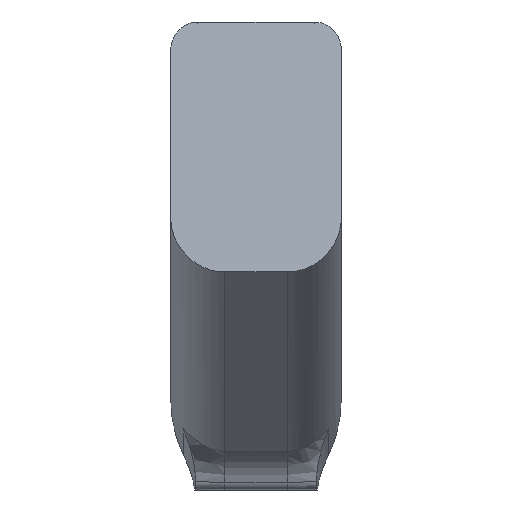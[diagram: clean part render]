
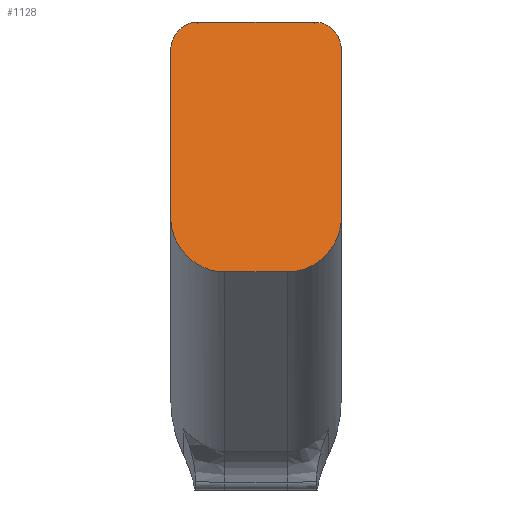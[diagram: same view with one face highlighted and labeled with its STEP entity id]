
A CAD part, front view. The second image highlights one B-rep face of the part: STEP entity #1128.
In plain terms, the highlighted planar face has unit normal (0, -0.978, 0.208).
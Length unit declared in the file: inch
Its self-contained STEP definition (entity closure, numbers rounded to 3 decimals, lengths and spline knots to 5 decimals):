
#7 = CARTESIAN_POINT ( 'NONE',  ( -0.22441, -2.64884, 0.92841 ) ) ;
#8 = CARTESIAN_POINT ( 'NONE',  ( -0.45503, -2.64884, 0.92841 ) ) ;
#15 = CARTESIAN_POINT ( 'NONE',  ( -0.61811, -2.56369, 1.32903 ) ) ;
#26 = CARTESIAN_POINT ( 'NONE',  ( -0.61811, -2.61357, 1.09436 ) ) ;
#27 = CARTESIAN_POINT ( 'NONE',  ( -0.61811, -2.64884, 0.92841 ) ) ;
#46 = DIRECTION ( 'NONE',  ( 0., -0.208, -0.978 ) ) ;
#50 = FACE_OUTER_BOUND ( 'NONE', #1464, .T. ) ;
#98 =( BOUNDED_CURVE ( )  B_SPLINE_CURVE ( 3, ( #1010, #1041, #1071, #1009 ),
 .UNSPECIFIED., .F., .F. ) 
 B_SPLINE_CURVE_WITH_KNOTS ( ( 4, 4 ),
 ( 4.71239, 6.28319 ),
 .UNSPECIFIED. ) 
 CURVE ( )  GEOMETRIC_REPRESENTATION_ITEM ( )  RATIONAL_B_SPLINE_CURVE ( ( 1., 0.805, 0.805, 1. ) ) 
 REPRESENTATION_ITEM ( '' )  );
#146 = CARTESIAN_POINT ( 'NONE',  ( -0.22441, -2.64884, 0.92841 ) ) ;
#226 = CARTESIAN_POINT ( 'NONE',  ( 0.61811, -2.26426, 2.73772 ) ) ;
#310 = VECTOR ( 'NONE', #1917, 39.37008 ) ;
#328 = VERTEX_POINT ( 'NONE', #146 ) ;
#376 = CARTESIAN_POINT ( 'NONE',  ( 0.61811, -2.56369, 1.32903 ) ) ;
#377 = CARTESIAN_POINT ( 'NONE',  ( 0.61811, -2.61357, 1.09436 ) ) ;
#386 = CARTESIAN_POINT ( 'NONE',  ( 0.22441, -2.64884, 0.92841 ) ) ;
#387 = CARTESIAN_POINT ( 'NONE',  ( 0.61811, -2.64884, 0.92841 ) ) ;
#431 = LINE ( 'NONE', #226, #2186 ) ;
#432 = DIRECTION ( 'NONE',  ( -1., 0., 0. ) ) ;
#433 = CARTESIAN_POINT ( 'NONE',  ( 0.45503, -2.64884, 0.92841 ) ) ;
#446 = VECTOR ( 'NONE', #46, 39.37008 ) ;
#468 = VERTEX_POINT ( 'NONE', #2005 ) ;
#499 = CARTESIAN_POINT ( 'NONE',  ( 0.42126, -2.26426, 2.73772 ) ) ;
#564 = VERTEX_POINT ( 'NONE', #1961 ) ;
#606 = VERTEX_POINT ( 'NONE', #1909 ) ;
#631 = AXIS2_PLACEMENT_3D ( 'NONE', #1594, #1531, #1529 ) ;
#782 = CARTESIAN_POINT ( 'NONE',  ( -0.61811, -2.30812, 2.53138 ) ) ;
#788 = CARTESIAN_POINT ( 'NONE',  ( -0.61811, -2.28243, 2.65225 ) ) ;
#791 = EDGE_CURVE ( 'NONE', #1135, #1896, #1317, .T. ) ;
#792 = DIRECTION ( 'NONE',  ( -1., 0., 0. ) ) ;
#811 = CARTESIAN_POINT ( 'NONE',  ( -0.42126, -2.26426, 2.73772 ) ) ;
#812 = CARTESIAN_POINT ( 'NONE',  ( -0.53657, -2.26426, 2.73772 ) ) ;
#911 = EDGE_CURVE ( 'NONE', #1135, #1552, #98, .T. ) ;
#947 = EDGE_CURVE ( 'NONE', #606, #468, #1353, .T. ) ;
#1009 = CARTESIAN_POINT ( 'NONE',  ( 0.42126, -2.26426, 2.73772 ) ) ;
#1010 = CARTESIAN_POINT ( 'NONE',  ( 0.61811, -2.30812, 2.53138 ) ) ;
#1041 = CARTESIAN_POINT ( 'NONE',  ( 0.61811, -2.28243, 2.65225 ) ) ;
#1071 = CARTESIAN_POINT ( 'NONE',  ( 0.53657, -2.26426, 2.73772 ) ) ;
#1128 = ADVANCED_FACE ( 'NONE', ( #50 ), #1557, .F. ) ;
#1135 = VERTEX_POINT ( 'NONE', #1566 ) ;
#1201 = ORIENTED_EDGE ( 'NONE', *, *, #1382, .T. ) ;
#1246 = CARTESIAN_POINT ( 'NONE',  ( -0.61811, -2.56369, 1.32903 ) ) ;
#1317 = LINE ( 'NONE', #1588, #310 ) ;
#1353 =( BOUNDED_CURVE ( )  B_SPLINE_CURVE ( 3, ( #811, #812, #788, #782 ),
 .UNSPECIFIED., .F., .F. ) 
 B_SPLINE_CURVE_WITH_KNOTS ( ( 4, 4 ),
 ( 3.14159, 4.71239 ),
 .UNSPECIFIED. ) 
 CURVE ( )  GEOMETRIC_REPRESENTATION_ITEM ( )  RATIONAL_B_SPLINE_CURVE ( ( 1., 0.805, 0.805, 1. ) ) 
 REPRESENTATION_ITEM ( '' )  );
#1366 = CARTESIAN_POINT ( 'NONE',  ( 0.61811, -2.56369, 1.32903 ) ) ;
#1380 = ORIENTED_EDGE ( 'NONE', *, *, #791, .F. ) ;
#1382 = EDGE_CURVE ( 'NONE', #1552, #606, #431, .T. ) ;
#1445 = ORIENTED_EDGE ( 'NONE', *, *, #1614, .F. ) ;
#1464 = EDGE_LOOP ( 'NONE', ( #1380, #1904, #1201, #2105, #1517, #1822, #1445, #1995 ) ) ;
#1517 = ORIENTED_EDGE ( 'NONE', *, *, #1779, .T. ) ;
#1529 = DIRECTION ( 'NONE',  ( 0., 0.208, 0.978 ) ) ;
#1531 = DIRECTION ( 'NONE',  ( 0., 0.978, -0.208 ) ) ;
#1539 = LINE ( 'NONE', #387, #1781 ) ;
#1552 = VERTEX_POINT ( 'NONE', #499 ) ;
#1557 = PLANE ( 'NONE',  #631 ) ;
#1566 = CARTESIAN_POINT ( 'NONE',  ( 0.61811, -2.30812, 2.53138 ) ) ;
#1588 = CARTESIAN_POINT ( 'NONE',  ( 0.61811, -2.64884, 0.92841 ) ) ;
#1594 = CARTESIAN_POINT ( 'NONE',  ( 0.61811, -2.64884, 0.92841 ) ) ;
#1600 = EDGE_CURVE ( 'NONE', #564, #1896, #1915, .T. ) ;
#1614 = EDGE_CURVE ( 'NONE', #564, #328, #1539, .T. ) ;
#1656 =( BOUNDED_CURVE ( )  B_SPLINE_CURVE ( 3, ( #15, #26, #8, #7 ),
 .UNSPECIFIED., .F., .T. ) 
 B_SPLINE_CURVE_WITH_KNOTS ( ( 4, 4 ),
 ( 1.5708, 3.14159 ),
 .UNSPECIFIED. ) 
 CURVE ( )  GEOMETRIC_REPRESENTATION_ITEM ( )  RATIONAL_B_SPLINE_CURVE ( ( 1., 0.805, 0.805, 1. ) ) 
 REPRESENTATION_ITEM ( '' )  );
#1779 = EDGE_CURVE ( 'NONE', #468, #1802, #1853, .T. ) ;
#1781 = VECTOR ( 'NONE', #432, 39.37008 ) ;
#1793 = EDGE_CURVE ( 'NONE', #1802, #328, #1656, .T. ) ;
#1802 = VERTEX_POINT ( 'NONE', #1246 ) ;
#1822 = ORIENTED_EDGE ( 'NONE', *, *, #1793, .T. ) ;
#1853 = LINE ( 'NONE', #27, #446 ) ;
#1896 = VERTEX_POINT ( 'NONE', #1366 ) ;
#1904 = ORIENTED_EDGE ( 'NONE', *, *, #911, .T. ) ;
#1909 = CARTESIAN_POINT ( 'NONE',  ( -0.42126, -2.26426, 2.73772 ) ) ;
#1915 =( BOUNDED_CURVE ( )  B_SPLINE_CURVE ( 3, ( #386, #433, #377, #376 ),
 .UNSPECIFIED., .F., .F. ) 
 B_SPLINE_CURVE_WITH_KNOTS ( ( 4, 4 ),
 ( 0., 1.5708 ),
 .UNSPECIFIED. ) 
 CURVE ( )  GEOMETRIC_REPRESENTATION_ITEM ( )  RATIONAL_B_SPLINE_CURVE ( ( 1., 0.805, 0.805, 1. ) ) 
 REPRESENTATION_ITEM ( '' )  );
#1917 = DIRECTION ( 'NONE',  ( 0., -0.208, -0.978 ) ) ;
#1961 = CARTESIAN_POINT ( 'NONE',  ( 0.22441, -2.64884, 0.92841 ) ) ;
#1995 = ORIENTED_EDGE ( 'NONE', *, *, #1600, .T. ) ;
#2005 = CARTESIAN_POINT ( 'NONE',  ( -0.61811, -2.30812, 2.53138 ) ) ;
#2105 = ORIENTED_EDGE ( 'NONE', *, *, #947, .T. ) ;
#2186 = VECTOR ( 'NONE', #792, 39.37008 ) ;
